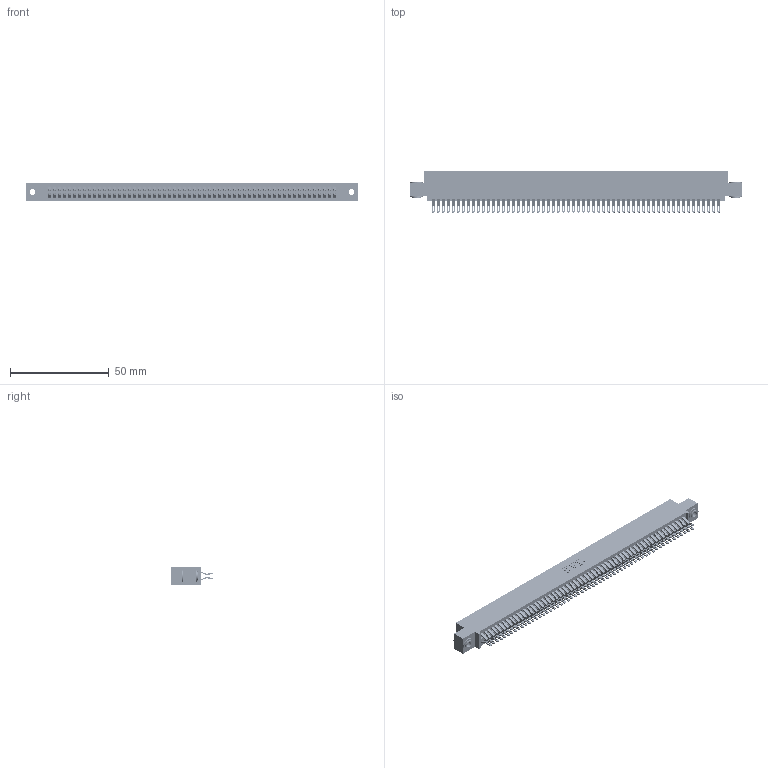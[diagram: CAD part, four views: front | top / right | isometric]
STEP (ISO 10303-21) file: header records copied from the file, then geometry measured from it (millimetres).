
FILE_DESCRIPTION (( 'STEP AP203' ), '1' );
FILE_NAME ('395-116-555-503.STEP', '2019-10-27T21:54:07', ( '' ), ( '' ), 'SwSTEP 2.0', 'SolidWorks 2016', '' );
FILE_SCHEMA (( 'CONFIG_CONTROL_DESIGN' ));
Length unit declared in the file: inch
Products named in the file (4): 345 Part_0.110 Offset - 0.156 Dia-TH; 345-292-001_555 Tail; 345-250-002_345-250-002-102; 395-116-555-503
Assembly tree (119 placements, depth 2):
  395-116-555-503
    345 Part_0.110 Offset - 0.156 Dia-TH
    345-292-001_555 Tail  x116
    345-250-002_345-250-002-102  x2
Bounding box: 168.53 x 21.13 x 9.4 mm (x, y, z)
Volume: 16802.1 mm3; surface area: 26614.2 mm2
Topology: 119 solids, 119 shells, 6664 faces, 20961 edges, 13970 vertices
Faces by surface type: plane 3690, cylinder 2966, cone 8
Entity records: 44462 total; most frequent: CARTESIAN_POINT 7449, ORIENTED_EDGE 7346, DIRECTION 6547, EDGE_CURVE 3673, LINE 3265, VECTOR 3265, VERTEX_POINT 2446, AXIS2_PLACEMENT_3D 1641
